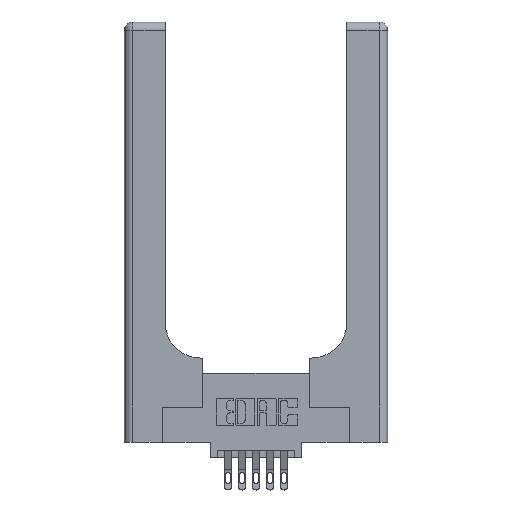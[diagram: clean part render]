
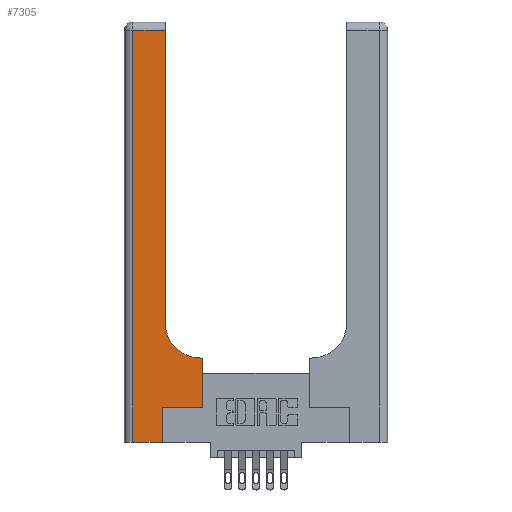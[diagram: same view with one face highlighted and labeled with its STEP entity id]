
A CAD part, top view. The second image highlights one B-rep face of the part: STEP entity #7305.
In plain terms, the highlighted planar face has unit normal (0, 0, 1).
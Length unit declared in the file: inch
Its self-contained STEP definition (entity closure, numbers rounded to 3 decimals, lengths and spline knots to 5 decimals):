
#175 = CARTESIAN_POINT ( 'NONE',  ( 0.269, 0., 0.37 ) ) ;
#670 = DIRECTION ( 'NONE',  ( 1., 0., 0. ) ) ;
#721 = CARTESIAN_POINT ( 'NONE',  ( 0.06, 2.94, 0.37 ) ) ;
#919 = EDGE_LOOP ( 'NONE', ( #12997, #932, #1819, #8114, #13849, #3490, #3347, #1534, #2847 ) ) ;
#932 = ORIENTED_EDGE ( 'NONE', *, *, #9626, .T. ) ;
#1051 = VERTEX_POINT ( 'NONE', #8496 ) ;
#1099 = DIRECTION ( 'NONE',  ( 0., 1., 0. ) ) ;
#1138 = EDGE_CURVE ( 'NONE', #7208, #11045, #14533, .T. ) ;
#1289 = CIRCLE ( 'NONE', #11227, 0.25 ) ;
#1318 = EDGE_CURVE ( 'NONE', #11045, #11723, #11705, .T. ) ;
#1534 = ORIENTED_EDGE ( 'NONE', *, *, #6704, .T. ) ;
#1744 = CARTESIAN_POINT ( 'NONE',  ( 0.5415, 0.6, 0.37 ) ) ;
#1819 = ORIENTED_EDGE ( 'NONE', *, *, #9735, .T. ) ;
#1890 = VECTOR ( 'NONE', #12196, 39.37008 ) ;
#2532 = VECTOR ( 'NONE', #7233, 39.37008 ) ;
#2847 = ORIENTED_EDGE ( 'NONE', *, *, #13118, .T. ) ;
#2989 = LINE ( 'NONE', #10137, #12091 ) ;
#3049 = CARTESIAN_POINT ( 'NONE',  ( 0.5585, 0.25, 0.37 ) ) ;
#3193 = CARTESIAN_POINT ( 'NONE',  ( 0.269, 0.25, 0.37 ) ) ;
#3347 = ORIENTED_EDGE ( 'NONE', *, *, #1318, .T. ) ;
#3490 = ORIENTED_EDGE ( 'NONE', *, *, #1138, .T. ) ;
#3996 = DIRECTION ( 'NONE',  ( 0., 0., -1. ) ) ;
#4006 = CARTESIAN_POINT ( 'NONE',  ( 0., 3., 0.37 ) ) ;
#4550 = VECTOR ( 'NONE', #11023, 39.37008 ) ;
#4716 = CARTESIAN_POINT ( 'NONE',  ( 0.06, 0., 0.37 ) ) ;
#6704 = EDGE_CURVE ( 'NONE', #11723, #7457, #2989, .T. ) ;
#7034 = DIRECTION ( 'NONE',  ( 0., 1., 0. ) ) ;
#7075 = VECTOR ( 'NONE', #1099, 39.37008 ) ;
#7208 = VERTEX_POINT ( 'NONE', #8254 ) ;
#7233 = DIRECTION ( 'NONE',  ( 0., 1., 0. ) ) ;
#7305 = ADVANCED_FACE ( 'NONE', ( #7551 ), #13998, .F. ) ;
#7457 = VERTEX_POINT ( 'NONE', #1744 ) ;
#7551 = FACE_OUTER_BOUND ( 'NONE', #919, .T. ) ;
#7610 = VECTOR ( 'NONE', #670, 39.37008 ) ;
#7635 = VERTEX_POINT ( 'NONE', #4716 ) ;
#7902 = EDGE_CURVE ( 'NONE', #7635, #10715, #8315, .T. ) ;
#7936 = VERTEX_POINT ( 'NONE', #721 ) ;
#7991 = CARTESIAN_POINT ( 'NONE',  ( 0.06, 3., 0.37 ) ) ;
#8108 = CARTESIAN_POINT ( 'NONE',  ( 0.5585, 0.6, 0.37 ) ) ;
#8114 = ORIENTED_EDGE ( 'NONE', *, *, #7902, .T. ) ;
#8245 = CARTESIAN_POINT ( 'NONE',  ( 0.2915, 2.94, 0.37 ) ) ;
#8254 = CARTESIAN_POINT ( 'NONE',  ( 0.269, 0.25, 0.37 ) ) ;
#8315 = LINE ( 'NONE', #12761, #7610 ) ;
#8496 = CARTESIAN_POINT ( 'NONE',  ( 0.2915, 0.85, 0.37 ) ) ;
#8608 = CARTESIAN_POINT ( 'NONE',  ( 0.5415, 0.85, 0.37 ) ) ;
#9169 = VERTEX_POINT ( 'NONE', #8245 ) ;
#9596 = LINE ( 'NONE', #7991, #14197 ) ;
#9626 = EDGE_CURVE ( 'NONE', #9169, #7936, #13667, .T. ) ;
#9735 = EDGE_CURVE ( 'NONE', #7936, #7635, #9596, .T. ) ;
#9751 = AXIS2_PLACEMENT_3D ( 'NONE', #4006, #11826, #13151 ) ;
#9798 = LINE ( 'NONE', #14380, #7075 ) ;
#10043 = CARTESIAN_POINT ( 'NONE',  ( 0., 2.94, 0.37 ) ) ;
#10137 = CARTESIAN_POINT ( 'NONE',  ( 0.2915, 0.6, 0.37 ) ) ;
#10285 = DIRECTION ( 'NONE',  ( 0., -1., 0. ) ) ;
#10715 = VERTEX_POINT ( 'NONE', #175 ) ;
#11023 = DIRECTION ( 'NONE',  ( -1., 0., 0. ) ) ;
#11045 = VERTEX_POINT ( 'NONE', #3049 ) ;
#11154 = CARTESIAN_POINT ( 'NONE',  ( 0.5585, 0.25, 0.37 ) ) ;
#11227 = AXIS2_PLACEMENT_3D ( 'NONE', #8608, #3996, #12920 ) ;
#11282 = DIRECTION ( 'NONE',  ( -1., 0., 0. ) ) ;
#11611 = CARTESIAN_POINT ( 'NONE',  ( 0.2915, 3., 0.37 ) ) ;
#11705 = LINE ( 'NONE', #11154, #14007 ) ;
#11723 = VERTEX_POINT ( 'NONE', #8108 ) ;
#11826 = DIRECTION ( 'NONE',  ( 0., 0., -1. ) ) ;
#11946 = LINE ( 'NONE', #11611, #2532 ) ;
#12091 = VECTOR ( 'NONE', #11282, 39.37008 ) ;
#12196 = DIRECTION ( 'NONE',  ( 1., 0., 0. ) ) ;
#12761 = CARTESIAN_POINT ( 'NONE',  ( 0., 0., 0.37 ) ) ;
#12920 = DIRECTION ( 'NONE',  ( 1., 0., 0. ) ) ;
#12972 = EDGE_CURVE ( 'NONE', #1051, #9169, #11946, .T. ) ;
#12997 = ORIENTED_EDGE ( 'NONE', *, *, #12972, .T. ) ;
#13118 = EDGE_CURVE ( 'NONE', #7457, #1051, #1289, .T. ) ;
#13151 = DIRECTION ( 'NONE',  ( -1., 0., 0. ) ) ;
#13667 = LINE ( 'NONE', #10043, #4550 ) ;
#13849 = ORIENTED_EDGE ( 'NONE', *, *, #13885, .T. ) ;
#13885 = EDGE_CURVE ( 'NONE', #10715, #7208, #9798, .T. ) ;
#13998 = PLANE ( 'NONE',  #9751 ) ;
#14007 = VECTOR ( 'NONE', #7034, 39.37008 ) ;
#14197 = VECTOR ( 'NONE', #10285, 39.37008 ) ;
#14380 = CARTESIAN_POINT ( 'NONE',  ( 0.269, 0., 0.37 ) ) ;
#14533 = LINE ( 'NONE', #3193, #1890 ) ;
